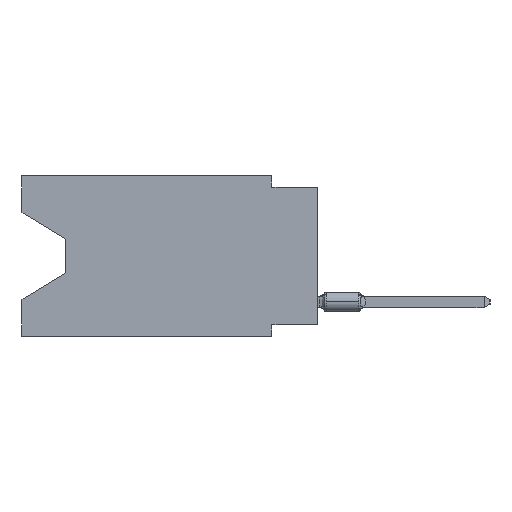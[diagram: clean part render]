
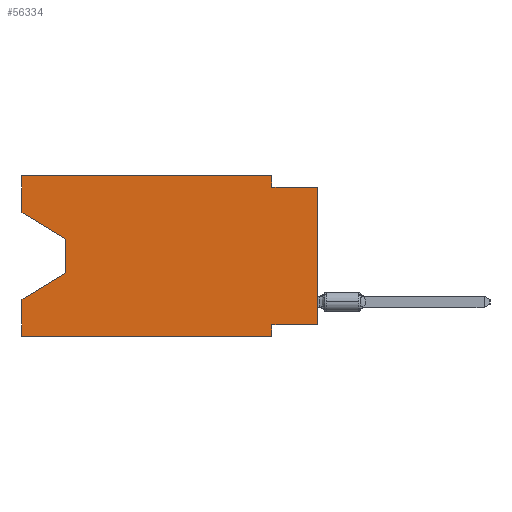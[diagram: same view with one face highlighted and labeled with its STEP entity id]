
A CAD part, left-side view. The second image highlights one B-rep face of the part: STEP entity #56334.
In plain terms, the highlighted planar face has unit normal (-1, 0, 0).
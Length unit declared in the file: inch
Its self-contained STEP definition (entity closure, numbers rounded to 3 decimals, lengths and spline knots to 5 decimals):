
#90 = VECTOR ( 'NONE', #40759, 39.37008 ) ;
#193 = ORIENTED_EDGE ( 'NONE', *, *, #49757, .T. ) ;
#493 = FACE_OUTER_BOUND ( 'NONE', #63210, .T. ) ;
#1767 = VECTOR ( 'NONE', #70909, 39.37008 ) ;
#2237 = PLANE ( 'NONE',  #16147 ) ;
#2477 = VERTEX_POINT ( 'NONE', #18990 ) ;
#2677 = EDGE_CURVE ( 'NONE', #60870, #65529, #27824, .T. ) ;
#2923 = VECTOR ( 'NONE', #33288, 39.37008 ) ;
#4596 = ORIENTED_EDGE ( 'NONE', *, *, #23879, .T. ) ;
#5017 = LINE ( 'NONE', #65636, #45960 ) ;
#6227 = VECTOR ( 'NONE', #70283, 39.37008 ) ;
#6311 = CARTESIAN_POINT ( 'NONE',  ( 0., 0.55, -0.212 ) ) ;
#7694 = EDGE_CURVE ( 'NONE', #21857, #15945, #31349, .T. ) ;
#8842 = VECTOR ( 'NONE', #31997, 39.37008 ) ;
#9143 = EDGE_CURVE ( 'NONE', #60870, #72024, #39884, .T. ) ;
#9483 = DIRECTION ( 'NONE',  ( 0., 0., -1. ) ) ;
#10664 = VECTOR ( 'NONE', #66665, 39.37008 ) ;
#10723 = LINE ( 'NONE', #17773, #1767 ) ;
#10790 = CARTESIAN_POINT ( 'NONE',  ( 0., 0.1, -0.35 ) ) ;
#15534 = VECTOR ( 'NONE', #9483, 39.37008 ) ;
#15945 = VERTEX_POINT ( 'NONE', #76324 ) ;
#16147 = AXIS2_PLACEMENT_3D ( 'NONE', #27464, #54476, #75732 ) ;
#16394 = ORIENTED_EDGE ( 'NONE', *, *, #23435, .F. ) ;
#16565 = CARTESIAN_POINT ( 'NONE',  ( 0., 0.55, -0.138 ) ) ;
#17773 = CARTESIAN_POINT ( 'NONE',  ( 0., 0.1, 0. ) ) ;
#18505 = DIRECTION ( 'NONE',  ( 0., 0., 1. ) ) ;
#18990 = CARTESIAN_POINT ( 'NONE',  ( 0., 0.1, -0.35 ) ) ;
#19178 = CARTESIAN_POINT ( 'NONE',  ( 0., 0.645, -0.26975 ) ) ;
#21290 = ORIENTED_EDGE ( 'NONE', *, *, #41336, .F. ) ;
#21857 = VERTEX_POINT ( 'NONE', #53277 ) ;
#23086 = LINE ( 'NONE', #50137, #53442 ) ;
#23435 = EDGE_CURVE ( 'NONE', #83776, #52163, #10723, .T. ) ;
#23879 = EDGE_CURVE ( 'NONE', #38279, #2477, #43526, .T. ) ;
#26732 = VERTEX_POINT ( 'NONE', #16565 ) ;
#27464 = CARTESIAN_POINT ( 'NONE',  ( 0., 0.645, 0. ) ) ;
#27824 = LINE ( 'NONE', #54837, #6227 ) ;
#28957 = CARTESIAN_POINT ( 'NONE',  ( 0., 0.1, 0. ) ) ;
#30086 = EDGE_CURVE ( 'NONE', #21857, #26732, #33106, .T. ) ;
#31333 = CARTESIAN_POINT ( 'NONE',  ( 0., 0.55, -0.212 ) ) ;
#31349 = LINE ( 'NONE', #86719, #72728 ) ;
#31694 = CARTESIAN_POINT ( 'NONE',  ( 0., 0.55, -0.138 ) ) ;
#31977 = DIRECTION ( 'NONE',  ( 0., -1., 0. ) ) ;
#31997 = DIRECTION ( 'NONE',  ( 0., -1., 0. ) ) ;
#33106 = LINE ( 'NONE', #73414, #78679 ) ;
#33288 = DIRECTION ( 'NONE',  ( 0., 0.855, -0.519 ) ) ;
#38279 = VERTEX_POINT ( 'NONE', #51206 ) ;
#38334 = EDGE_CURVE ( 'NONE', #38279, #81111, #84003, .T. ) ;
#39884 = LINE ( 'NONE', #66897, #90 ) ;
#40759 = DIRECTION ( 'NONE',  ( 0., 1., 0. ) ) ;
#41336 = EDGE_CURVE ( 'NONE', #72024, #2477, #51076, .T. ) ;
#43037 = DIRECTION ( 'NONE',  ( 0., -1., 0. ) ) ;
#43526 = LINE ( 'NONE', #59881, #8842 ) ;
#43849 = ORIENTED_EDGE ( 'NONE', *, *, #61493, .F. ) ;
#44728 = ORIENTED_EDGE ( 'NONE', *, *, #77933, .T. ) ;
#45278 = ORIENTED_EDGE ( 'NONE', *, *, #38334, .F. ) ;
#45960 = VECTOR ( 'NONE', #31977, 39.37008 ) ;
#47008 = LINE ( 'NONE', #6311, #2923 ) ;
#49757 = EDGE_CURVE ( 'NONE', #83196, #81111, #47008, .T. ) ;
#50137 = CARTESIAN_POINT ( 'NONE',  ( 0., 0., -0.025 ) ) ;
#51076 = LINE ( 'NONE', #10790, #15534 ) ;
#51206 = CARTESIAN_POINT ( 'NONE',  ( 0., 0.645, -0.35 ) ) ;
#52163 = VERTEX_POINT ( 'NONE', #87190 ) ;
#52897 = ORIENTED_EDGE ( 'NONE', *, *, #2677, .T. ) ;
#52957 = LINE ( 'NONE', #31694, #10664 ) ;
#53277 = CARTESIAN_POINT ( 'NONE',  ( 0., 0.645, -0.08025 ) ) ;
#53442 = VECTOR ( 'NONE', #43037, 39.37008 ) ;
#54476 = DIRECTION ( 'NONE',  ( 1., 0., 0. ) ) ;
#54837 = CARTESIAN_POINT ( 'NONE',  ( 0., 0., 0. ) ) ;
#56334 = ADVANCED_FACE ( 'NONE', ( #493 ), #2237, .F. ) ;
#58850 = CARTESIAN_POINT ( 'NONE',  ( 0., 0., -0.325 ) ) ;
#59881 = CARTESIAN_POINT ( 'NONE',  ( 0., 0.645, -0.35 ) ) ;
#60870 = VERTEX_POINT ( 'NONE', #58850 ) ;
#61493 = EDGE_CURVE ( 'NONE', #52163, #65529, #23086, .T. ) ;
#62203 = ORIENTED_EDGE ( 'NONE', *, *, #7694, .F. ) ;
#63210 = EDGE_LOOP ( 'NONE', ( #64412, #44728, #193, #45278, #4596, #21290, #65622, #52897, #43849, #16394, #68661, #62203 ) ) ;
#64412 = ORIENTED_EDGE ( 'NONE', *, *, #30086, .T. ) ;
#65529 = VERTEX_POINT ( 'NONE', #66154 ) ;
#65622 = ORIENTED_EDGE ( 'NONE', *, *, #9143, .F. ) ;
#65636 = CARTESIAN_POINT ( 'NONE',  ( 0., 0.645, 0. ) ) ;
#66154 = CARTESIAN_POINT ( 'NONE',  ( 0., 0., -0.025 ) ) ;
#66665 = DIRECTION ( 'NONE',  ( 0., 0., -1. ) ) ;
#66897 = CARTESIAN_POINT ( 'NONE',  ( 0., 0., -0.325 ) ) ;
#68661 = ORIENTED_EDGE ( 'NONE', *, *, #74316, .F. ) ;
#70283 = DIRECTION ( 'NONE',  ( 0., 0., 1. ) ) ;
#70909 = DIRECTION ( 'NONE',  ( 0., 0., -1. ) ) ;
#71997 = CARTESIAN_POINT ( 'NONE',  ( 0., 0.645, 0. ) ) ;
#72024 = VERTEX_POINT ( 'NONE', #85300 ) ;
#72728 = VECTOR ( 'NONE', #18505, 39.37008 ) ;
#73414 = CARTESIAN_POINT ( 'NONE',  ( 0., 0.645, -0.08025 ) ) ;
#74316 = EDGE_CURVE ( 'NONE', #15945, #83776, #5017, .T. ) ;
#75732 = DIRECTION ( 'NONE',  ( 0., 0., -1. ) ) ;
#76324 = CARTESIAN_POINT ( 'NONE',  ( 0., 0.645, 0. ) ) ;
#77933 = EDGE_CURVE ( 'NONE', #26732, #83196, #52957, .T. ) ;
#78679 = VECTOR ( 'NONE', #84217, 39.37008 ) ;
#79056 = VECTOR ( 'NONE', #85316, 39.37008 ) ;
#81111 = VERTEX_POINT ( 'NONE', #19178 ) ;
#83196 = VERTEX_POINT ( 'NONE', #31333 ) ;
#83776 = VERTEX_POINT ( 'NONE', #28957 ) ;
#84003 = LINE ( 'NONE', #71997, #79056 ) ;
#84217 = DIRECTION ( 'NONE',  ( 0., -0.855, -0.519 ) ) ;
#85300 = CARTESIAN_POINT ( 'NONE',  ( 0., 0.1, -0.325 ) ) ;
#85316 = DIRECTION ( 'NONE',  ( 0., 0., 1. ) ) ;
#86719 = CARTESIAN_POINT ( 'NONE',  ( 0., 0.645, 0. ) ) ;
#87190 = CARTESIAN_POINT ( 'NONE',  ( 0., 0.1, -0.025 ) ) ;
